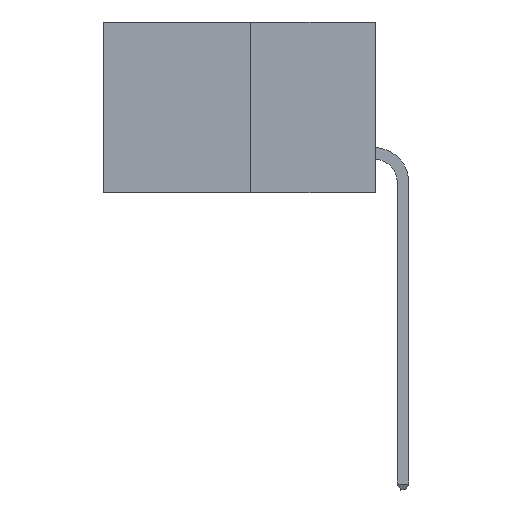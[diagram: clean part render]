
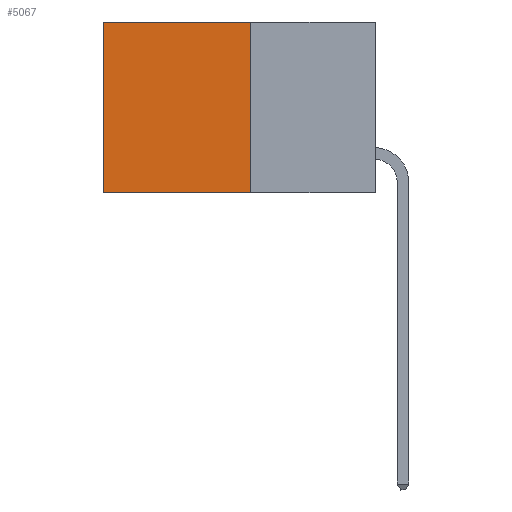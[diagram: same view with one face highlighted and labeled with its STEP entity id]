
A CAD part, left-side view. The second image highlights one B-rep face of the part: STEP entity #5067.
In plain terms, the highlighted planar face has unit normal (-1, 0, 0).
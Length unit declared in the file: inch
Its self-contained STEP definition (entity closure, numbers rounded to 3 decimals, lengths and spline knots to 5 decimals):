
#113 = ORIENTED_EDGE ( 'NONE', *, *, #5788, .T. ) ;
#257 = DIRECTION ( 'NONE',  ( 1., 0., 0. ) ) ;
#374 = ORIENTED_EDGE ( 'NONE', *, *, #711, .F. ) ;
#558 = VECTOR ( 'NONE', #6508, 39.37008 ) ;
#711 = EDGE_CURVE ( 'NONE', #10651, #8209, #13347, .T. ) ;
#1088 = CARTESIAN_POINT ( 'NONE',  ( 0.277, 0.27, -0.37 ) ) ;
#1975 = FACE_OUTER_BOUND ( 'NONE', #6159, .T. ) ;
#3009 = CARTESIAN_POINT ( 'NONE',  ( 0.277, 0.27, -0.37 ) ) ;
#3354 = ORIENTED_EDGE ( 'NONE', *, *, #6578, .F. ) ;
#4283 = AXIS2_PLACEMENT_3D ( 'NONE', #8851, #257, #8903 ) ;
#4545 = VECTOR ( 'NONE', #8273, 39.37008 ) ;
#4554 = LINE ( 'NONE', #4612, #7410 ) ;
#4612 = CARTESIAN_POINT ( 'NONE',  ( 0.277, 0.59, -0.37 ) ) ;
#4921 = LINE ( 'NONE', #1088, #5302 ) ;
#5067 = ADVANCED_FACE ( 'NONE', ( #1975 ), #14748, .F. ) ;
#5280 = CARTESIAN_POINT ( 'NONE',  ( 0.277, 0.27, 0. ) ) ;
#5302 = VECTOR ( 'NONE', #9723, 39.37008 ) ;
#5788 = EDGE_CURVE ( 'NONE', #13668, #14377, #4554, .T. ) ;
#5865 = DIRECTION ( 'NONE',  ( 0., 0., -1. ) ) ;
#6159 = EDGE_LOOP ( 'NONE', ( #113, #3354, #374, #7030 ) ) ;
#6508 = DIRECTION ( 'NONE',  ( 0., 1., 0. ) ) ;
#6578 = EDGE_CURVE ( 'NONE', #8209, #14377, #4921, .T. ) ;
#7030 = ORIENTED_EDGE ( 'NONE', *, *, #9752, .T. ) ;
#7410 = VECTOR ( 'NONE', #5865, 39.37008 ) ;
#8146 = CARTESIAN_POINT ( 'NONE',  ( 0.277, 0.59, -0.37 ) ) ;
#8209 = VERTEX_POINT ( 'NONE', #3009 ) ;
#8273 = DIRECTION ( 'NONE',  ( 0., 0., -1. ) ) ;
#8829 = CARTESIAN_POINT ( 'NONE',  ( 0.277, 0.27, -0.37 ) ) ;
#8851 = CARTESIAN_POINT ( 'NONE',  ( 0.277, 0.27, -0.37 ) ) ;
#8903 = DIRECTION ( 'NONE',  ( 0., 0., -1. ) ) ;
#9723 = DIRECTION ( 'NONE',  ( 0., 1., 0. ) ) ;
#9752 = EDGE_CURVE ( 'NONE', #10651, #13668, #15448, .T. ) ;
#10444 = CARTESIAN_POINT ( 'NONE',  ( 0.277, 0.59, 0. ) ) ;
#10651 = VERTEX_POINT ( 'NONE', #15218 ) ;
#13347 = LINE ( 'NONE', #8829, #4545 ) ;
#13668 = VERTEX_POINT ( 'NONE', #10444 ) ;
#14377 = VERTEX_POINT ( 'NONE', #8146 ) ;
#14748 = PLANE ( 'NONE',  #4283 ) ;
#15218 = CARTESIAN_POINT ( 'NONE',  ( 0.277, 0.27, 0. ) ) ;
#15448 = LINE ( 'NONE', #5280, #558 ) ;
